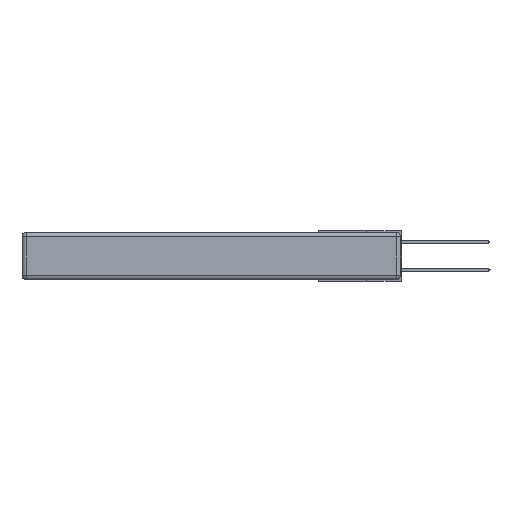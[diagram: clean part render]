
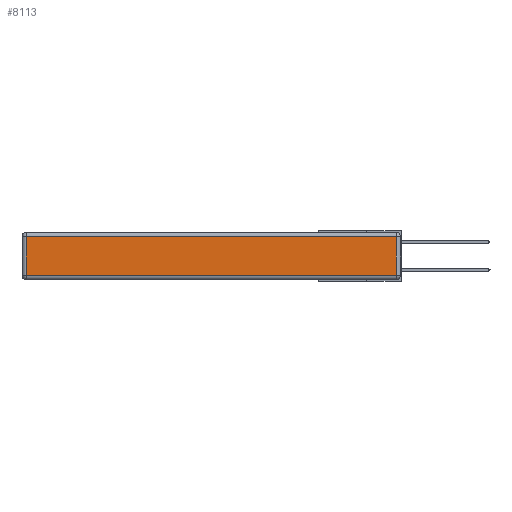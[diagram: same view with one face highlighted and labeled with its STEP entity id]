
A CAD part, left-side view. The second image highlights one B-rep face of the part: STEP entity #8113.
In plain terms, the highlighted planar face has unit normal (-1, 0, 0).
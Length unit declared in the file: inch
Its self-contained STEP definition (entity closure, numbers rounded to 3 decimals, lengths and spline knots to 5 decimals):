
#406 = CARTESIAN_POINT ( 'NONE',  ( 0., 2.72, -0.343 ) ) ;
#1141 = CARTESIAN_POINT ( 'NONE',  ( 0., 2.72, -0.03 ) ) ;
#1306 = LINE ( 'NONE', #23816, #21862 ) ;
#2158 = CARTESIAN_POINT ( 'NONE',  ( 0., 0.03, -0.03 ) ) ;
#2667 = DIRECTION ( 'NONE',  ( 0., -1., 0. ) ) ;
#3068 = EDGE_LOOP ( 'NONE', ( #19815, #19088, #5018, #16092 ) ) ;
#5018 = ORIENTED_EDGE ( 'NONE', *, *, #24142, .T. ) ;
#5623 = AXIS2_PLACEMENT_3D ( 'NONE', #20202, #9697, #18374 ) ;
#6919 = EDGE_CURVE ( 'NONE', #23047, #16629, #13554, .T. ) ;
#8113 = ADVANCED_FACE ( 'NONE', ( #10419 ), #20554, .T. ) ;
#8560 = DIRECTION ( 'NONE',  ( 0., 0., -1. ) ) ;
#8789 = CARTESIAN_POINT ( 'NONE',  ( 0., 0.03, -0.313 ) ) ;
#9697 = DIRECTION ( 'NONE',  ( -1., 0., 0. ) ) ;
#10419 = FACE_OUTER_BOUND ( 'NONE', #3068, .T. ) ;
#13554 = LINE ( 'NONE', #23700, #26959 ) ;
#16092 = ORIENTED_EDGE ( 'NONE', *, *, #24081, .T. ) ;
#16629 = VERTEX_POINT ( 'NONE', #8789 ) ;
#17648 = VERTEX_POINT ( 'NONE', #1141 ) ;
#18374 = DIRECTION ( 'NONE',  ( 0., 0., 1. ) ) ;
#19076 = DIRECTION ( 'NONE',  ( 0., 1., 0. ) ) ;
#19088 = ORIENTED_EDGE ( 'NONE', *, *, #20794, .T. ) ;
#19815 = ORIENTED_EDGE ( 'NONE', *, *, #6919, .T. ) ;
#20116 = CARTESIAN_POINT ( 'NONE',  ( 0., 0.03, -0.343 ) ) ;
#20202 = CARTESIAN_POINT ( 'NONE',  ( 0., 0., -0.343 ) ) ;
#20470 = DIRECTION ( 'NONE',  ( 0., 0., 1. ) ) ;
#20539 = LINE ( 'NONE', #406, #21521 ) ;
#20554 = PLANE ( 'NONE',  #5623 ) ;
#20794 = EDGE_CURVE ( 'NONE', #16629, #21191, #21670, .T. ) ;
#21191 = VERTEX_POINT ( 'NONE', #2158 ) ;
#21521 = VECTOR ( 'NONE', #8560, 39.37008 ) ;
#21670 = LINE ( 'NONE', #20116, #24269 ) ;
#21862 = VECTOR ( 'NONE', #19076, 39.37008 ) ;
#23047 = VERTEX_POINT ( 'NONE', #26403 ) ;
#23700 = CARTESIAN_POINT ( 'NONE',  ( 0., 0., -0.313 ) ) ;
#23816 = CARTESIAN_POINT ( 'NONE',  ( 0., 2.75, -0.03 ) ) ;
#24081 = EDGE_CURVE ( 'NONE', #17648, #23047, #20539, .T. ) ;
#24142 = EDGE_CURVE ( 'NONE', #21191, #17648, #1306, .T. ) ;
#24269 = VECTOR ( 'NONE', #20470, 39.37008 ) ;
#26403 = CARTESIAN_POINT ( 'NONE',  ( 0., 2.72, -0.313 ) ) ;
#26959 = VECTOR ( 'NONE', #2667, 39.37008 ) ;
